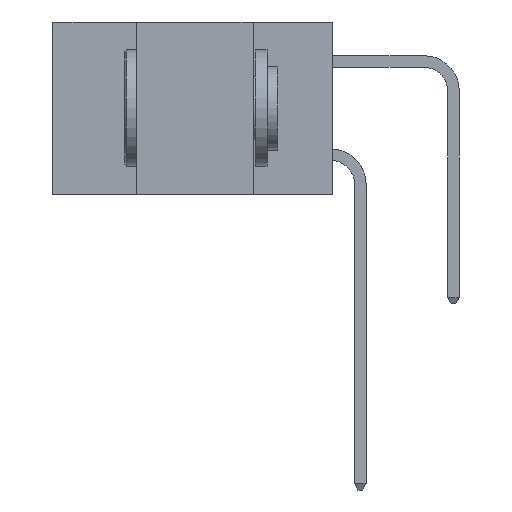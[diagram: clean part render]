
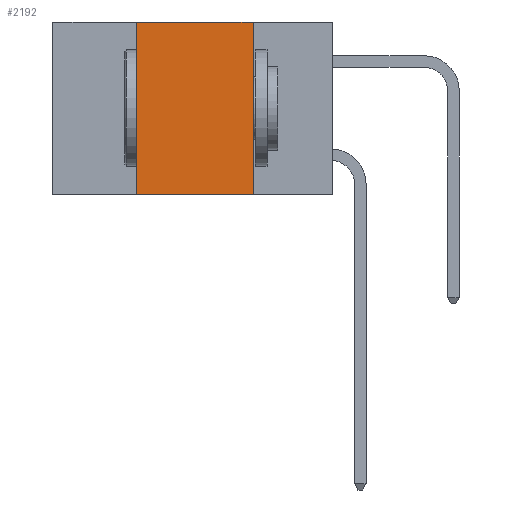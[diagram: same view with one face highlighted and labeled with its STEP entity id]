
A CAD part, left-side view. The second image highlights one B-rep face of the part: STEP entity #2192.
In plain terms, the highlighted planar face has unit normal (-1, 0, 0).
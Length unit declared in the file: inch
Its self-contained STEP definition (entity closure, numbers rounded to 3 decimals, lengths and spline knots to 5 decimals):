
#400 = VECTOR ( 'NONE', #9111, 39.37008 ) ;
#1387 = VERTEX_POINT ( 'NONE', #7020 ) ;
#1388 = LINE ( 'NONE', #11058, #13219 ) ;
#1529 = VERTEX_POINT ( 'NONE', #5121 ) ;
#2192 = ADVANCED_FACE ( 'NONE', ( #14406 ), #14332, .F. ) ;
#2949 = DIRECTION ( 'NONE',  ( 1., 0., 0. ) ) ;
#3282 = DIRECTION ( 'NONE',  ( 0., -1., 0. ) ) ;
#3430 = CARTESIAN_POINT ( 'NONE',  ( 0., 0.6, -0.37 ) ) ;
#5041 = CARTESIAN_POINT ( 'NONE',  ( 0., 0.42, 0. ) ) ;
#5121 = CARTESIAN_POINT ( 'NONE',  ( 0., 0.17, 0. ) ) ;
#5167 = ORIENTED_EDGE ( 'NONE', *, *, #5606, .F. ) ;
#5220 = EDGE_CURVE ( 'NONE', #8644, #1387, #6548, .T. ) ;
#5606 = EDGE_CURVE ( 'NONE', #1529, #1387, #10139, .T. ) ;
#6548 = LINE ( 'NONE', #3430, #13376 ) ;
#6558 = ORIENTED_EDGE ( 'NONE', *, *, #5220, .T. ) ;
#6663 = VERTEX_POINT ( 'NONE', #5041 ) ;
#6722 = CARTESIAN_POINT ( 'NONE',  ( 0., 0.6, 0. ) ) ;
#7020 = CARTESIAN_POINT ( 'NONE',  ( 0., 0.17, -0.37 ) ) ;
#7520 = ORIENTED_EDGE ( 'NONE', *, *, #11867, .F. ) ;
#8340 = AXIS2_PLACEMENT_3D ( 'NONE', #6722, #2949, #11644 ) ;
#8644 = VERTEX_POINT ( 'NONE', #14604 ) ;
#9025 = CARTESIAN_POINT ( 'NONE',  ( 0., 0.17, -0.37 ) ) ;
#9111 = DIRECTION ( 'NONE',  ( 0., 0., -1. ) ) ;
#9233 = EDGE_LOOP ( 'NONE', ( #5167, #13162, #7520, #6558 ) ) ;
#10139 = LINE ( 'NONE', #9025, #400 ) ;
#10952 = VECTOR ( 'NONE', #11811, 39.37008 ) ;
#11058 = CARTESIAN_POINT ( 'NONE',  ( 0., 0.6, 0. ) ) ;
#11644 = DIRECTION ( 'NONE',  ( 0., 0., -1. ) ) ;
#11811 = DIRECTION ( 'NONE',  ( 0., 0., 1. ) ) ;
#11867 = EDGE_CURVE ( 'NONE', #8644, #6663, #14163, .T. ) ;
#12138 = EDGE_CURVE ( 'NONE', #6663, #1529, #1388, .T. ) ;
#12969 = CARTESIAN_POINT ( 'NONE',  ( 0., 0.42, -0.37 ) ) ;
#13162 = ORIENTED_EDGE ( 'NONE', *, *, #12138, .F. ) ;
#13219 = VECTOR ( 'NONE', #14682, 39.37008 ) ;
#13376 = VECTOR ( 'NONE', #3282, 39.37008 ) ;
#14163 = LINE ( 'NONE', #12969, #10952 ) ;
#14332 = PLANE ( 'NONE',  #8340 ) ;
#14406 = FACE_OUTER_BOUND ( 'NONE', #9233, .T. ) ;
#14604 = CARTESIAN_POINT ( 'NONE',  ( 0., 0.42, -0.37 ) ) ;
#14682 = DIRECTION ( 'NONE',  ( 0., -1., 0. ) ) ;
